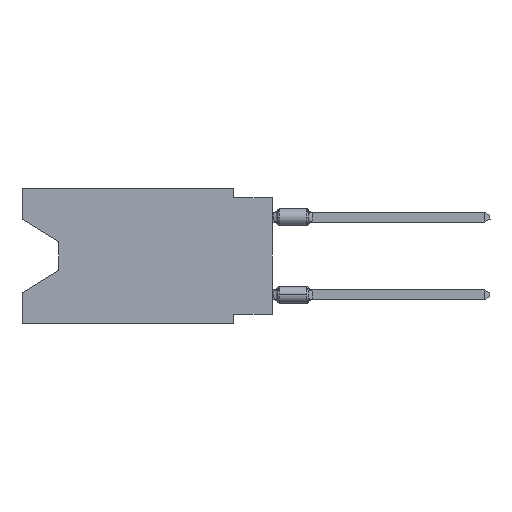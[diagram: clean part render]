
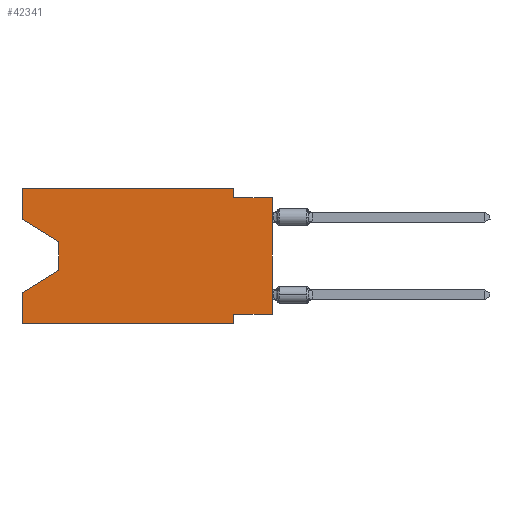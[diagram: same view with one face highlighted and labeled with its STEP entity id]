
A CAD part, left-side view. The second image highlights one B-rep face of the part: STEP entity #42341.
In plain terms, the highlighted planar face has unit normal (-1, 0, 0).
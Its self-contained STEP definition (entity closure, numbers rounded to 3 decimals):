
#222 = CARTESIAN_POINT ( 'NONE',  ( 0., 0., -8.255 ) ) ;
#1742 = VECTOR ( 'NONE', #40087, 1000. ) ;
#1984 = LINE ( 'NONE', #37282, #25802 ) ;
#2056 = EDGE_CURVE ( 'NONE', #26490, #39653, #31898, .T. ) ;
#2069 = DIRECTION ( 'NONE',  ( 0., 0., -1. ) ) ;
#2253 = EDGE_LOOP ( 'NONE', ( #2921, #16926, #14348, #44973, #8320, #3446, #21781, #21317, #15718, #33830, #31554, #20049 ) ) ;
#2528 = VECTOR ( 'NONE', #31492, 1000. ) ;
#2657 = VECTOR ( 'NONE', #2069, 1000. ) ;
#2921 = ORIENTED_EDGE ( 'NONE', *, *, #47047, .T. ) ;
#3165 = CARTESIAN_POINT ( 'NONE',  ( 0., 16.383, -8.89 ) ) ;
#3243 = LINE ( 'NONE', #46002, #36314 ) ;
#3446 = ORIENTED_EDGE ( 'NONE', *, *, #9262, .F. ) ;
#3815 = VECTOR ( 'NONE', #27028, 1000. ) ;
#4343 = CARTESIAN_POINT ( 'NONE',  ( 0., 13.97, -5.385 ) ) ;
#5990 = VERTEX_POINT ( 'NONE', #13778 ) ;
#6756 = LINE ( 'NONE', #41301, #12811 ) ;
#7209 = CARTESIAN_POINT ( 'NONE',  ( 0., 2.54, -8.255 ) ) ;
#7431 = EDGE_CURVE ( 'NONE', #48876, #8321, #43444, .T. ) ;
#8320 = ORIENTED_EDGE ( 'NONE', *, *, #19466, .T. ) ;
#8321 = VERTEX_POINT ( 'NONE', #14325 ) ;
#9262 = EDGE_CURVE ( 'NONE', #27202, #41853, #6756, .T. ) ;
#9550 = VERTEX_POINT ( 'NONE', #25383 ) ;
#9936 = DIRECTION ( 'NONE',  ( 0., 0., 1. ) ) ;
#10293 = LINE ( 'NONE', #35270, #18409 ) ;
#11803 = CARTESIAN_POINT ( 'NONE',  ( 0., 0., -0.635 ) ) ;
#12057 = LINE ( 'NONE', #11803, #2528 ) ;
#12584 = VECTOR ( 'NONE', #29052, 1000. ) ;
#12671 = EDGE_CURVE ( 'NONE', #13357, #39653, #12057, .T. ) ;
#12811 = VECTOR ( 'NONE', #33115, 1000. ) ;
#13357 = VERTEX_POINT ( 'NONE', #26019 ) ;
#13460 = LINE ( 'NONE', #41077, #12584 ) ;
#13778 = CARTESIAN_POINT ( 'NONE',  ( 0., 16.383, -2.038 ) ) ;
#14103 = CARTESIAN_POINT ( 'NONE',  ( 0., 13.97, -3.505 ) ) ;
#14125 = DIRECTION ( 'NONE',  ( 0., 0., -1. ) ) ;
#14202 = AXIS2_PLACEMENT_3D ( 'NONE', #19452, #19196, #19706 ) ;
#14325 = CARTESIAN_POINT ( 'NONE',  ( 0., 16.383, -6.852 ) ) ;
#14348 = ORIENTED_EDGE ( 'NONE', *, *, #7431, .T. ) ;
#14368 = EDGE_CURVE ( 'NONE', #9550, #13357, #10293, .T. ) ;
#14728 = EDGE_CURVE ( 'NONE', #5990, #48309, #1984, .T. ) ;
#15005 = LINE ( 'NONE', #30608, #3815 ) ;
#15107 = PLANE ( 'NONE',  #14202 ) ;
#15718 = ORIENTED_EDGE ( 'NONE', *, *, #12671, .F. ) ;
#16541 = CARTESIAN_POINT ( 'NONE',  ( 0., 0., 0. ) ) ;
#16926 = ORIENTED_EDGE ( 'NONE', *, *, #40974, .T. ) ;
#18025 = LINE ( 'NONE', #3165, #40614 ) ;
#18372 = VERTEX_POINT ( 'NONE', #28176 ) ;
#18409 = VECTOR ( 'NONE', #14125, 1000. ) ;
#18854 = DIRECTION ( 'NONE',  ( 0., -0.855, -0.519 ) ) ;
#19002 = EDGE_CURVE ( 'NONE', #18372, #8321, #15005, .T. ) ;
#19196 = DIRECTION ( 'NONE',  ( 1., 0., 0. ) ) ;
#19452 = CARTESIAN_POINT ( 'NONE',  ( 0., 16.383, 0. ) ) ;
#19466 = EDGE_CURVE ( 'NONE', #18372, #41853, #18025, .T. ) ;
#19706 = DIRECTION ( 'NONE',  ( 0., 0., -1. ) ) ;
#19743 = CARTESIAN_POINT ( 'NONE',  ( 0., 16.383, 0. ) ) ;
#20049 = ORIENTED_EDGE ( 'NONE', *, *, #14728, .F. ) ;
#21317 = ORIENTED_EDGE ( 'NONE', *, *, #2056, .T. ) ;
#21781 = ORIENTED_EDGE ( 'NONE', *, *, #46139, .F. ) ;
#22688 = CARTESIAN_POINT ( 'NONE',  ( 0., 16.383, 0. ) ) ;
#22837 = VECTOR ( 'NONE', #32399, 1000. ) ;
#24981 = CARTESIAN_POINT ( 'NONE',  ( 0., 13.97, -5.385 ) ) ;
#25361 = LINE ( 'NONE', #14103, #2657 ) ;
#25383 = CARTESIAN_POINT ( 'NONE',  ( 0., 2.54, 0. ) ) ;
#25748 = CARTESIAN_POINT ( 'NONE',  ( 0., 2.54, -8.89 ) ) ;
#25802 = VECTOR ( 'NONE', #9936, 1000. ) ;
#26019 = CARTESIAN_POINT ( 'NONE',  ( 0., 2.54, -0.635 ) ) ;
#26490 = VERTEX_POINT ( 'NONE', #222 ) ;
#27028 = DIRECTION ( 'NONE',  ( 0., 0., 1. ) ) ;
#27044 = DIRECTION ( 'NONE',  ( 0., -1., 0. ) ) ;
#27142 = VECTOR ( 'NONE', #27044, 1000. ) ;
#27202 = VERTEX_POINT ( 'NONE', #7209 ) ;
#28176 = CARTESIAN_POINT ( 'NONE',  ( 0., 16.383, -8.89 ) ) ;
#29052 = DIRECTION ( 'NONE',  ( 0., 1., 0. ) ) ;
#29455 = VERTEX_POINT ( 'NONE', #34994 ) ;
#30608 = CARTESIAN_POINT ( 'NONE',  ( 0., 16.383, 0. ) ) ;
#31492 = DIRECTION ( 'NONE',  ( 0., -1., 0. ) ) ;
#31554 = ORIENTED_EDGE ( 'NONE', *, *, #38927, .F. ) ;
#31898 = LINE ( 'NONE', #16541, #1742 ) ;
#32399 = DIRECTION ( 'NONE',  ( 0., 0.855, -0.519 ) ) ;
#33115 = DIRECTION ( 'NONE',  ( 0., 0., -1. ) ) ;
#33830 = ORIENTED_EDGE ( 'NONE', *, *, #14368, .F. ) ;
#34199 = LINE ( 'NONE', #22688, #27142 ) ;
#34994 = CARTESIAN_POINT ( 'NONE',  ( 0., 13.97, -3.505 ) ) ;
#35270 = CARTESIAN_POINT ( 'NONE',  ( 0., 2.54, 0. ) ) ;
#36314 = VECTOR ( 'NONE', #18854, 1000. ) ;
#37282 = CARTESIAN_POINT ( 'NONE',  ( 0., 16.383, 0. ) ) ;
#38647 = FACE_OUTER_BOUND ( 'NONE', #2253, .T. ) ;
#38927 = EDGE_CURVE ( 'NONE', #48309, #9550, #34199, .T. ) ;
#39653 = VERTEX_POINT ( 'NONE', #48482 ) ;
#40087 = DIRECTION ( 'NONE',  ( 0., 0., 1. ) ) ;
#40614 = VECTOR ( 'NONE', #49272, 1000. ) ;
#40974 = EDGE_CURVE ( 'NONE', #29455, #48876, #25361, .T. ) ;
#41077 = CARTESIAN_POINT ( 'NONE',  ( 0., 0., -8.255 ) ) ;
#41301 = CARTESIAN_POINT ( 'NONE',  ( 0., 2.54, -8.89 ) ) ;
#41853 = VERTEX_POINT ( 'NONE', #25748 ) ;
#42341 = ADVANCED_FACE ( 'NONE', ( #38647 ), #15107, .F. ) ;
#43444 = LINE ( 'NONE', #24981, #22837 ) ;
#44973 = ORIENTED_EDGE ( 'NONE', *, *, #19002, .F. ) ;
#46002 = CARTESIAN_POINT ( 'NONE',  ( 0., 16.383, -2.038 ) ) ;
#46139 = EDGE_CURVE ( 'NONE', #26490, #27202, #13460, .T. ) ;
#47047 = EDGE_CURVE ( 'NONE', #5990, #29455, #3243, .T. ) ;
#48309 = VERTEX_POINT ( 'NONE', #19743 ) ;
#48482 = CARTESIAN_POINT ( 'NONE',  ( 0., 0., -0.635 ) ) ;
#48876 = VERTEX_POINT ( 'NONE', #4343 ) ;
#49272 = DIRECTION ( 'NONE',  ( 0., -1., 0. ) ) ;
